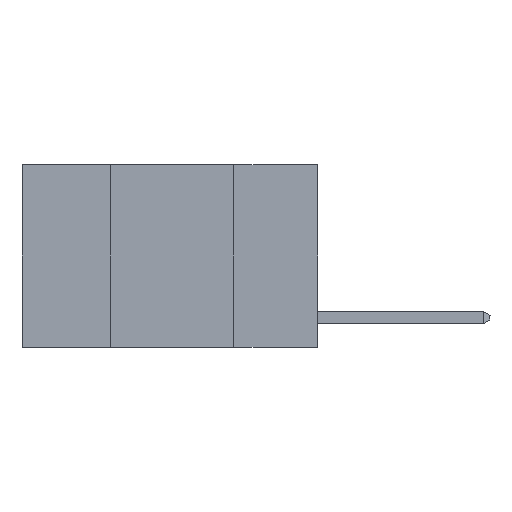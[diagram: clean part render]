
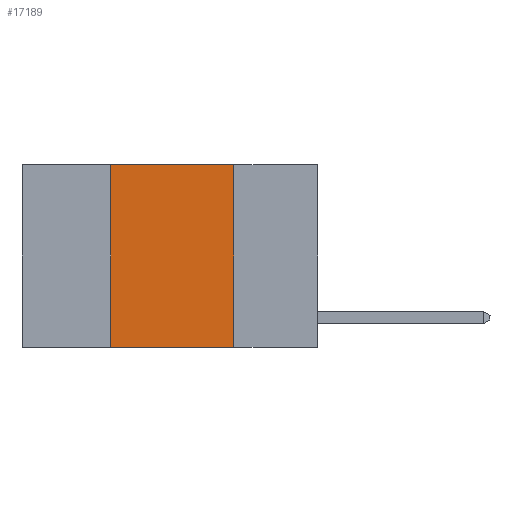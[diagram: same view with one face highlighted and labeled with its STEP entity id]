
A CAD part, left-side view. The second image highlights one B-rep face of the part: STEP entity #17189.
In plain terms, the highlighted planar face has unit normal (-1, 0, 0).
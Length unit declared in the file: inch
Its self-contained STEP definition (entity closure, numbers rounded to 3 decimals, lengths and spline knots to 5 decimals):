
#306 = ORIENTED_EDGE ( 'NONE', *, *, #13863, .F. ) ;
#701 = VERTEX_POINT ( 'NONE', #11747 ) ;
#2333 = DIRECTION ( 'NONE',  ( 0., 0., -1. ) ) ;
#2568 = DIRECTION ( 'NONE',  ( 0., 0., -1. ) ) ;
#3181 = DIRECTION ( 'NONE',  ( 0., -1., 0. ) ) ;
#3742 = CARTESIAN_POINT ( 'NONE',  ( 0., 0.42, 0. ) ) ;
#3952 = EDGE_LOOP ( 'NONE', ( #17885, #306, #6512, #12020 ) ) ;
#5730 = LINE ( 'NONE', #13898, #15164 ) ;
#6512 = ORIENTED_EDGE ( 'NONE', *, *, #12736, .F. ) ;
#6795 = VECTOR ( 'NONE', #3181, 39.37008 ) ;
#9192 = CARTESIAN_POINT ( 'NONE',  ( 0., 0.6, -0.37 ) ) ;
#10812 = VECTOR ( 'NONE', #22420, 39.37008 ) ;
#11390 = LINE ( 'NONE', #9192, #10812 ) ;
#11477 = EDGE_CURVE ( 'NONE', #24494, #19088, #11390, .T. ) ;
#11709 = CARTESIAN_POINT ( 'NONE',  ( 0., 0.42, -0.37 ) ) ;
#11747 = CARTESIAN_POINT ( 'NONE',  ( 0., 0.42, 0. ) ) ;
#11756 = CARTESIAN_POINT ( 'NONE',  ( 0., 0.6, 0. ) ) ;
#11778 = LINE ( 'NONE', #20125, #6795 ) ;
#12020 = ORIENTED_EDGE ( 'NONE', *, *, #11477, .T. ) ;
#12736 = EDGE_CURVE ( 'NONE', #24494, #701, #22851, .T. ) ;
#13666 = DIRECTION ( 'NONE',  ( 1., 0., 0. ) ) ;
#13863 = EDGE_CURVE ( 'NONE', #701, #18844, #11778, .T. ) ;
#13898 = CARTESIAN_POINT ( 'NONE',  ( 0., 0.17, 0. ) ) ;
#15109 = CARTESIAN_POINT ( 'NONE',  ( 0., 0.17, 0. ) ) ;
#15164 = VECTOR ( 'NONE', #2568, 39.37008 ) ;
#17189 = ADVANCED_FACE ( 'NONE', ( #19901 ), #23038, .F. ) ;
#17795 = EDGE_CURVE ( 'NONE', #18844, #19088, #5730, .T. ) ;
#17862 = VECTOR ( 'NONE', #18885, 39.37008 ) ;
#17885 = ORIENTED_EDGE ( 'NONE', *, *, #17795, .F. ) ;
#18844 = VERTEX_POINT ( 'NONE', #15109 ) ;
#18885 = DIRECTION ( 'NONE',  ( 0., 0., 1. ) ) ;
#19088 = VERTEX_POINT ( 'NONE', #19556 ) ;
#19556 = CARTESIAN_POINT ( 'NONE',  ( 0., 0.17, -0.37 ) ) ;
#19901 = FACE_OUTER_BOUND ( 'NONE', #3952, .T. ) ;
#20125 = CARTESIAN_POINT ( 'NONE',  ( 0., 0.6, 0. ) ) ;
#20878 = AXIS2_PLACEMENT_3D ( 'NONE', #11756, #13666, #2333 ) ;
#22420 = DIRECTION ( 'NONE',  ( 0., -1., 0. ) ) ;
#22851 = LINE ( 'NONE', #3742, #17862 ) ;
#23038 = PLANE ( 'NONE',  #20878 ) ;
#24494 = VERTEX_POINT ( 'NONE', #11709 ) ;
